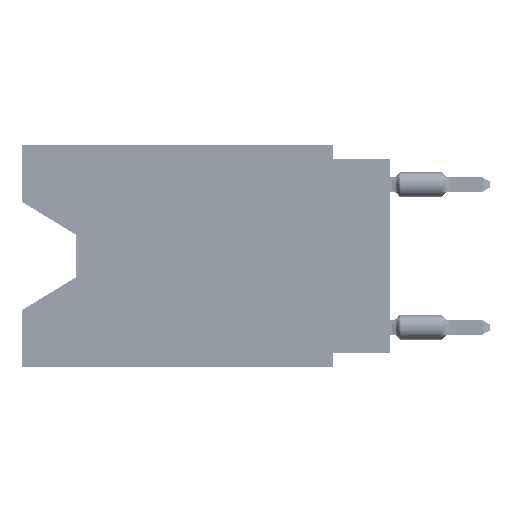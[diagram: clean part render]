
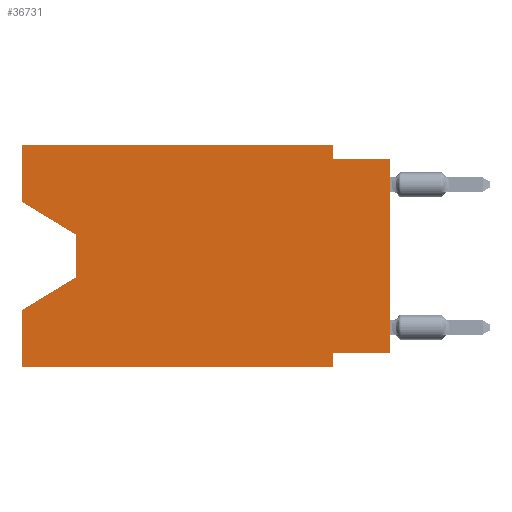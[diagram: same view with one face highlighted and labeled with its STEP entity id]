
A CAD part, left-side view. The second image highlights one B-rep face of the part: STEP entity #36731.
In plain terms, the highlighted planar face has unit normal (-1, 0, 0).
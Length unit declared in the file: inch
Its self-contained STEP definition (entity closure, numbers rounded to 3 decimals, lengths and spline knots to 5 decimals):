
#123 = VERTEX_POINT ( 'NONE', #57449 ) ;
#2637 = VECTOR ( 'NONE', #44362, 39.37008 ) ;
#3934 = DIRECTION ( 'NONE',  ( 0., 0., 1. ) ) ;
#4139 = EDGE_CURVE ( 'NONE', #25028, #56935, #64203, .T. ) ;
#4439 = CARTESIAN_POINT ( 'NONE',  ( 0., 0., -0.025 ) ) ;
#4804 = VECTOR ( 'NONE', #32349, 39.37008 ) ;
#6853 = CARTESIAN_POINT ( 'NONE',  ( 0., 0.1, -0.025 ) ) ;
#7769 = PLANE ( 'NONE',  #55781 ) ;
#7805 = ORIENTED_EDGE ( 'NONE', *, *, #42494, .T. ) ;
#8109 = CARTESIAN_POINT ( 'NONE',  ( 0., 0.645, -0.39 ) ) ;
#8326 = CARTESIAN_POINT ( 'NONE',  ( 0., 0.1, -0.39 ) ) ;
#9372 = ORIENTED_EDGE ( 'NONE', *, *, #42497, .T. ) ;
#10536 = ORIENTED_EDGE ( 'NONE', *, *, #83497, .F. ) ;
#13664 = EDGE_CURVE ( 'NONE', #69350, #123, #82621, .T. ) ;
#14162 = FACE_OUTER_BOUND ( 'NONE', #28386, .T. ) ;
#14389 = EDGE_CURVE ( 'NONE', #47102, #16813, #47422, .T. ) ;
#16813 = VERTEX_POINT ( 'NONE', #8326 ) ;
#17895 = CARTESIAN_POINT ( 'NONE',  ( 0., 0.645, 0. ) ) ;
#18309 = CARTESIAN_POINT ( 'NONE',  ( 0., 0.645, 0. ) ) ;
#18651 = DIRECTION ( 'NONE',  ( 0., 0., -1. ) ) ;
#20276 = ORIENTED_EDGE ( 'NONE', *, *, #13664, .F. ) ;
#20339 = VERTEX_POINT ( 'NONE', #39136 ) ;
#21430 = VECTOR ( 'NONE', #68321, 39.37008 ) ;
#21703 = CARTESIAN_POINT ( 'NONE',  ( 0., 0.1, -0.365 ) ) ;
#23821 = CARTESIAN_POINT ( 'NONE',  ( 0., 0.645, -0.10025 ) ) ;
#23879 = LINE ( 'NONE', #18309, #2637 ) ;
#24661 = DIRECTION ( 'NONE',  ( 0., -0.855, -0.519 ) ) ;
#25028 = VERTEX_POINT ( 'NONE', #51474 ) ;
#25134 = DIRECTION ( 'NONE',  ( 0., 1., 0. ) ) ;
#25291 = CARTESIAN_POINT ( 'NONE',  ( 0., 0., 0. ) ) ;
#26335 = CARTESIAN_POINT ( 'NONE',  ( 0., 0.1, -0.39 ) ) ;
#27196 = CARTESIAN_POINT ( 'NONE',  ( 0., 0., -0.365 ) ) ;
#27313 = LINE ( 'NONE', #79889, #46596 ) ;
#28012 = ORIENTED_EDGE ( 'NONE', *, *, #76585, .F. ) ;
#28386 = EDGE_LOOP ( 'NONE', ( #9372, #7805, #37543, #67774, #81538, #43764, #28012, #48208, #20276, #52154, #45439, #10536 ) ) ;
#30395 = CARTESIAN_POINT ( 'NONE',  ( 0., 0.645, 0. ) ) ;
#30481 = DIRECTION ( 'NONE',  ( 0., -1., 0. ) ) ;
#30627 = EDGE_CURVE ( 'NONE', #35865, #69350, #27313, .T. ) ;
#30761 = DIRECTION ( 'NONE',  ( 1., 0., 0. ) ) ;
#30931 = DIRECTION ( 'NONE',  ( 0., 0.855, -0.519 ) ) ;
#32349 = DIRECTION ( 'NONE',  ( 0., 0., -1. ) ) ;
#32423 = CARTESIAN_POINT ( 'NONE',  ( 0., 0.645, -0.28975 ) ) ;
#32958 = VERTEX_POINT ( 'NONE', #38539 ) ;
#35515 = DIRECTION ( 'NONE',  ( 0., 0., -1. ) ) ;
#35865 = VERTEX_POINT ( 'NONE', #70623 ) ;
#36731 = ADVANCED_FACE ( 'NONE', ( #14162 ), #7769, .F. ) ;
#37543 = ORIENTED_EDGE ( 'NONE', *, *, #4139, .T. ) ;
#38539 = CARTESIAN_POINT ( 'NONE',  ( 0., 0.645, 0. ) ) ;
#38743 = LINE ( 'NONE', #26335, #4804 ) ;
#39136 = CARTESIAN_POINT ( 'NONE',  ( 0., 0.645, -0.10025 ) ) ;
#42494 = EDGE_CURVE ( 'NONE', #78285, #25028, #55857, .T. ) ;
#42497 = EDGE_CURVE ( 'NONE', #20339, #78285, #82792, .T. ) ;
#43471 = CARTESIAN_POINT ( 'NONE',  ( 0., 0.55, -0.158 ) ) ;
#43637 = LINE ( 'NONE', #30395, #45930 ) ;
#43764 = ORIENTED_EDGE ( 'NONE', *, *, #47421, .F. ) ;
#43907 = VERTEX_POINT ( 'NONE', #27196 ) ;
#44362 = DIRECTION ( 'NONE',  ( 0., -1., 0. ) ) ;
#45439 = ORIENTED_EDGE ( 'NONE', *, *, #59635, .F. ) ;
#45930 = VECTOR ( 'NONE', #3934, 39.37008 ) ;
#46033 = CARTESIAN_POINT ( 'NONE',  ( 0., 0., -0.365 ) ) ;
#46596 = VECTOR ( 'NONE', #53380, 39.37008 ) ;
#46640 = EDGE_CURVE ( 'NONE', #43907, #123, #72258, .T. ) ;
#46683 = VECTOR ( 'NONE', #18651, 39.37008 ) ;
#47102 = VERTEX_POINT ( 'NONE', #8109 ) ;
#47421 = EDGE_CURVE ( 'NONE', #53254, #16813, #38743, .T. ) ;
#47422 = LINE ( 'NONE', #61483, #21430 ) ;
#48208 = ORIENTED_EDGE ( 'NONE', *, *, #46640, .T. ) ;
#51474 = CARTESIAN_POINT ( 'NONE',  ( 0., 0.55, -0.232 ) ) ;
#52154 = ORIENTED_EDGE ( 'NONE', *, *, #30627, .F. ) ;
#53254 = VERTEX_POINT ( 'NONE', #21703 ) ;
#53380 = DIRECTION ( 'NONE',  ( 0., 0., -1. ) ) ;
#53444 = CARTESIAN_POINT ( 'NONE',  ( 0., 0.645, 0. ) ) ;
#54056 = CARTESIAN_POINT ( 'NONE',  ( 0., 0.55, -0.158 ) ) ;
#55781 = AXIS2_PLACEMENT_3D ( 'NONE', #53444, #30761, #35515 ) ;
#55857 = LINE ( 'NONE', #43471, #46683 ) ;
#56123 = CARTESIAN_POINT ( 'NONE',  ( 0., 0.55, -0.232 ) ) ;
#56326 = LINE ( 'NONE', #17895, #76392 ) ;
#56935 = VERTEX_POINT ( 'NONE', #32423 ) ;
#57449 = CARTESIAN_POINT ( 'NONE',  ( 0., 0., -0.025 ) ) ;
#59635 = EDGE_CURVE ( 'NONE', #32958, #35865, #23879, .T. ) ;
#61483 = CARTESIAN_POINT ( 'NONE',  ( 0., 0.645, -0.39 ) ) ;
#64203 = LINE ( 'NONE', #56123, #70216 ) ;
#65409 = VECTOR ( 'NONE', #30481, 39.37008 ) ;
#67774 = ORIENTED_EDGE ( 'NONE', *, *, #76417, .F. ) ;
#67970 = LINE ( 'NONE', #46033, #83283 ) ;
#68321 = DIRECTION ( 'NONE',  ( 0., -1., 0. ) ) ;
#69350 = VERTEX_POINT ( 'NONE', #6853 ) ;
#70216 = VECTOR ( 'NONE', #30931, 39.37008 ) ;
#70623 = CARTESIAN_POINT ( 'NONE',  ( 0., 0.1, 0. ) ) ;
#72258 = LINE ( 'NONE', #25291, #78332 ) ;
#75600 = DIRECTION ( 'NONE',  ( 0., 0., 1. ) ) ;
#76392 = VECTOR ( 'NONE', #75600, 39.37008 ) ;
#76417 = EDGE_CURVE ( 'NONE', #47102, #56935, #56326, .T. ) ;
#76585 = EDGE_CURVE ( 'NONE', #43907, #53254, #67970, .T. ) ;
#78091 = VECTOR ( 'NONE', #24661, 39.37008 ) ;
#78285 = VERTEX_POINT ( 'NONE', #54056 ) ;
#78332 = VECTOR ( 'NONE', #78686, 39.37008 ) ;
#78686 = DIRECTION ( 'NONE',  ( 0., 0., 1. ) ) ;
#79889 = CARTESIAN_POINT ( 'NONE',  ( 0., 0.1, 0. ) ) ;
#81538 = ORIENTED_EDGE ( 'NONE', *, *, #14389, .T. ) ;
#82621 = LINE ( 'NONE', #4439, #65409 ) ;
#82792 = LINE ( 'NONE', #23821, #78091 ) ;
#83283 = VECTOR ( 'NONE', #25134, 39.37008 ) ;
#83497 = EDGE_CURVE ( 'NONE', #20339, #32958, #43637, .T. ) ;
